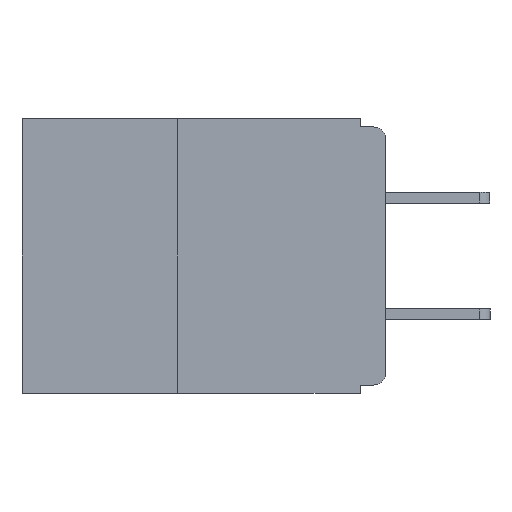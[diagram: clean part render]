
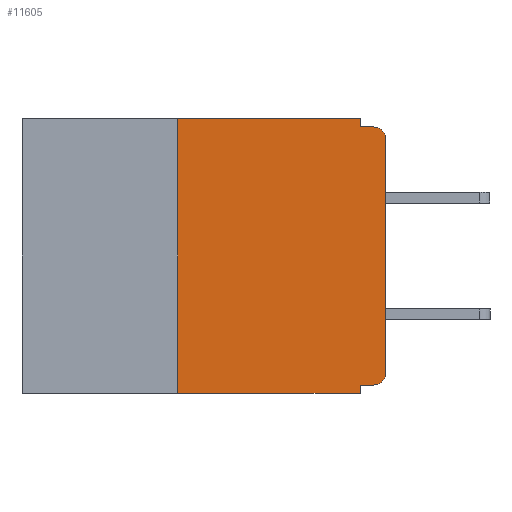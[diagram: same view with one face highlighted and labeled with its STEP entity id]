
A CAD part, left-side view. The second image highlights one B-rep face of the part: STEP entity #11605.
In plain terms, the highlighted planar face has unit normal (-1, 0, 0).
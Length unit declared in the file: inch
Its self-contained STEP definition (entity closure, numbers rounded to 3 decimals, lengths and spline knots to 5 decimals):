
#93 = DIRECTION ( 'NONE',  ( 0., -1., 0. ) ) ;
#232 = VECTOR ( 'NONE', #14350, 39.37008 ) ;
#249 = CARTESIAN_POINT ( 'NONE',  ( 0., 0.437, 0. ) ) ;
#320 = CARTESIAN_POINT ( 'NONE',  ( 0., 0., -0.01 ) ) ;
#400 = VERTEX_POINT ( 'NONE', #4874 ) ;
#454 = DIRECTION ( 'NONE',  ( -1., 0., 0. ) ) ;
#485 = EDGE_CURVE ( 'NONE', #400, #23392, #5368, .T. ) ;
#2075 = DIRECTION ( 'NONE',  ( 0., 0., 1. ) ) ;
#2170 = CARTESIAN_POINT ( 'NONE',  ( 0., 0.015, -0.01 ) ) ;
#2284 = DIRECTION ( 'NONE',  ( 1., 0., 0. ) ) ;
#2773 = CIRCLE ( 'NONE', #11508, 0.015 ) ;
#2829 = ORIENTED_EDGE ( 'NONE', *, *, #14952, .T. ) ;
#3744 = ORIENTED_EDGE ( 'NONE', *, *, #5550, .F. ) ;
#3973 = EDGE_CURVE ( 'NONE', #19245, #23392, #10715, .T. ) ;
#4753 = VECTOR ( 'NONE', #22724, 39.37008 ) ;
#4874 = CARTESIAN_POINT ( 'NONE',  ( 0., 0.031, -0.32 ) ) ;
#4959 = ORIENTED_EDGE ( 'NONE', *, *, #3973, .T. ) ;
#5034 = CARTESIAN_POINT ( 'NONE',  ( 0., 0.25, 0. ) ) ;
#5368 = LINE ( 'NONE', #23358, #4753 ) ;
#5550 = EDGE_CURVE ( 'NONE', #22977, #16702, #7363, .T. ) ;
#5816 = VERTEX_POINT ( 'NONE', #11625 ) ;
#6161 = EDGE_CURVE ( 'NONE', #19496, #400, #12768, .T. ) ;
#6399 = EDGE_CURVE ( 'NONE', #6539, #16702, #13044, .T. ) ;
#6539 = VERTEX_POINT ( 'NONE', #21821 ) ;
#7363 = LINE ( 'NONE', #320, #16917 ) ;
#7636 = VECTOR ( 'NONE', #9015, 39.37008 ) ;
#8650 = CARTESIAN_POINT ( 'NONE',  ( 0., 0.437, 0. ) ) ;
#8924 = LINE ( 'NONE', #11838, #24084 ) ;
#9015 = DIRECTION ( 'NONE',  ( 0., 1., 0. ) ) ;
#9232 = EDGE_CURVE ( 'NONE', #12522, #5816, #9327, .T. ) ;
#9327 = LINE ( 'NONE', #8650, #18834 ) ;
#9598 = CARTESIAN_POINT ( 'NONE',  ( 0., 0.25, -0.33 ) ) ;
#9888 = CARTESIAN_POINT ( 'NONE',  ( 0., 0.031, -0.01 ) ) ;
#9988 = CARTESIAN_POINT ( 'NONE',  ( 0., 0.015, -0.025 ) ) ;
#10715 = LINE ( 'NONE', #16230, #232 ) ;
#11508 = AXIS2_PLACEMENT_3D ( 'NONE', #12224, #454, #14123 ) ;
#11605 = ADVANCED_FACE ( 'NONE', ( #24979 ), #23387, .F. ) ;
#11625 = CARTESIAN_POINT ( 'NONE',  ( 0., 0.031, 0. ) ) ;
#11838 = CARTESIAN_POINT ( 'NONE',  ( 0., 0., 0. ) ) ;
#11937 = DIRECTION ( 'NONE',  ( 0., 0., -1. ) ) ;
#12224 = CARTESIAN_POINT ( 'NONE',  ( 0., 0.015, -0.305 ) ) ;
#12522 = VERTEX_POINT ( 'NONE', #5034 ) ;
#12768 = LINE ( 'NONE', #16599, #7636 ) ;
#12780 = VECTOR ( 'NONE', #17214, 39.37008 ) ;
#13044 = CIRCLE ( 'NONE', #24953, 0.015 ) ;
#14123 = DIRECTION ( 'NONE',  ( 0., 0., -1. ) ) ;
#14171 = CARTESIAN_POINT ( 'NONE',  ( 0., 0.015, -0.32 ) ) ;
#14350 = DIRECTION ( 'NONE',  ( 0., -1., 0. ) ) ;
#14705 = ORIENTED_EDGE ( 'NONE', *, *, #24762, .F. ) ;
#14848 = ORIENTED_EDGE ( 'NONE', *, *, #23709, .T. ) ;
#14952 = EDGE_CURVE ( 'NONE', #23175, #6539, #8924, .T. ) ;
#15332 = CARTESIAN_POINT ( 'NONE',  ( 0., 0.031, 0. ) ) ;
#15844 = DIRECTION ( 'NONE',  ( 0., 0., -1. ) ) ;
#16229 = VECTOR ( 'NONE', #20270, 39.37008 ) ;
#16230 = CARTESIAN_POINT ( 'NONE',  ( 0., 0.437, -0.33 ) ) ;
#16599 = CARTESIAN_POINT ( 'NONE',  ( 0., 0., -0.32 ) ) ;
#16702 = VERTEX_POINT ( 'NONE', #2170 ) ;
#16807 = LINE ( 'NONE', #18366, #16229 ) ;
#16917 = VECTOR ( 'NONE', #93, 39.37008 ) ;
#17214 = DIRECTION ( 'NONE',  ( 0., 0., -1. ) ) ;
#17883 = ORIENTED_EDGE ( 'NONE', *, *, #6399, .T. ) ;
#18211 = DIRECTION ( 'NONE',  ( 0., -1., 0. ) ) ;
#18366 = CARTESIAN_POINT ( 'NONE',  ( 0., 0.25, -0.33 ) ) ;
#18582 = ORIENTED_EDGE ( 'NONE', *, *, #485, .F. ) ;
#18834 = VECTOR ( 'NONE', #18211, 39.37008 ) ;
#19245 = VERTEX_POINT ( 'NONE', #9598 ) ;
#19496 = VERTEX_POINT ( 'NONE', #14171 ) ;
#20212 = EDGE_CURVE ( 'NONE', #19245, #12522, #16807, .T. ) ;
#20270 = DIRECTION ( 'NONE',  ( 0., 0., 1. ) ) ;
#20769 = CARTESIAN_POINT ( 'NONE',  ( 0., 0.031, -0.33 ) ) ;
#20785 = ORIENTED_EDGE ( 'NONE', *, *, #20212, .F. ) ;
#21821 = CARTESIAN_POINT ( 'NONE',  ( 0., 0., -0.025 ) ) ;
#22724 = DIRECTION ( 'NONE',  ( 0., 0., -1. ) ) ;
#22826 = LINE ( 'NONE', #15332, #12780 ) ;
#22977 = VERTEX_POINT ( 'NONE', #9888 ) ;
#23175 = VERTEX_POINT ( 'NONE', #23857 ) ;
#23302 = DIRECTION ( 'NONE',  ( -1., 0., 0. ) ) ;
#23358 = CARTESIAN_POINT ( 'NONE',  ( 0., 0.031, -0.33 ) ) ;
#23387 = PLANE ( 'NONE',  #23400 ) ;
#23392 = VERTEX_POINT ( 'NONE', #20769 ) ;
#23400 = AXIS2_PLACEMENT_3D ( 'NONE', #249, #2284, #15844 ) ;
#23709 = EDGE_CURVE ( 'NONE', #19496, #23175, #2773, .T. ) ;
#23857 = CARTESIAN_POINT ( 'NONE',  ( 0., 0., -0.305 ) ) ;
#23902 = ORIENTED_EDGE ( 'NONE', *, *, #9232, .F. ) ;
#24084 = VECTOR ( 'NONE', #2075, 39.37008 ) ;
#24568 = EDGE_LOOP ( 'NONE', ( #2829, #17883, #3744, #14705, #23902, #20785, #4959, #18582, #24891, #14848 ) ) ;
#24762 = EDGE_CURVE ( 'NONE', #5816, #22977, #22826, .T. ) ;
#24891 = ORIENTED_EDGE ( 'NONE', *, *, #6161, .F. ) ;
#24953 = AXIS2_PLACEMENT_3D ( 'NONE', #9988, #23302, #11937 ) ;
#24979 = FACE_OUTER_BOUND ( 'NONE', #24568, .T. ) ;
